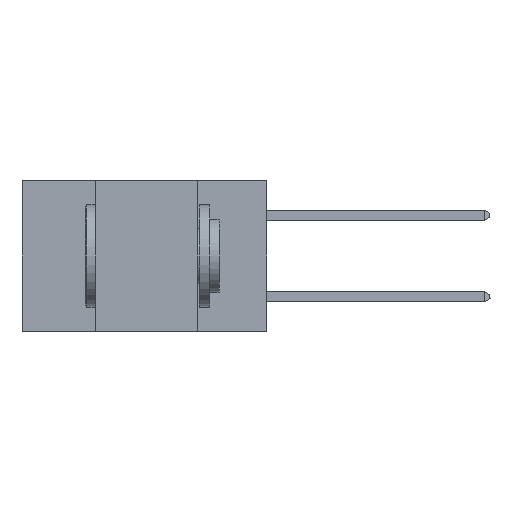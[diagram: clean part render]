
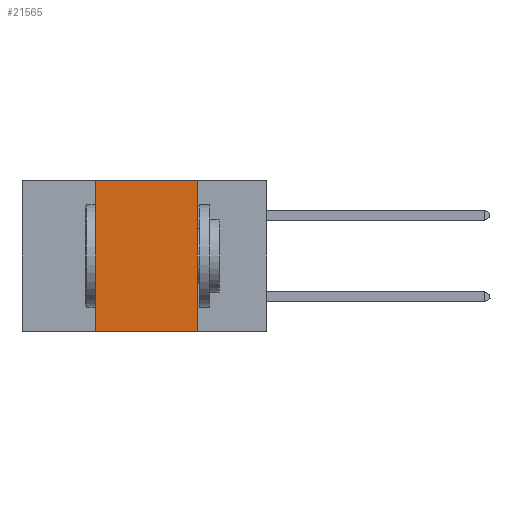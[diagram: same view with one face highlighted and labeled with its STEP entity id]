
A CAD part, left-side view. The second image highlights one B-rep face of the part: STEP entity #21565.
In plain terms, the highlighted planar face has unit normal (-1, 0, 0).
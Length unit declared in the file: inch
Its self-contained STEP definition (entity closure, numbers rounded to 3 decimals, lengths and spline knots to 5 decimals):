
#768 = DIRECTION ( 'NONE',  ( 0., -1., 0. ) ) ;
#1853 = VECTOR ( 'NONE', #768, 39.37008 ) ;
#1929 = ORIENTED_EDGE ( 'NONE', *, *, #16639, .F. ) ;
#1976 = LINE ( 'NONE', #21147, #2717 ) ;
#2556 = VERTEX_POINT ( 'NONE', #9746 ) ;
#2717 = VECTOR ( 'NONE', #15711, 39.37008 ) ;
#3177 = EDGE_CURVE ( 'NONE', #22099, #7793, #5542, .T. ) ;
#3540 = CARTESIAN_POINT ( 'NONE',  ( 0., 0.17, -0.37 ) ) ;
#3684 = LINE ( 'NONE', #7576, #5959 ) ;
#4507 = FACE_OUTER_BOUND ( 'NONE', #18668, .T. ) ;
#5542 = LINE ( 'NONE', #13347, #1853 ) ;
#5700 = CARTESIAN_POINT ( 'NONE',  ( 0., 0.6, 0. ) ) ;
#5959 = VECTOR ( 'NONE', #20226, 39.37008 ) ;
#6013 = DIRECTION ( 'NONE',  ( 0., 0., -1. ) ) ;
#7150 = VECTOR ( 'NONE', #7552, 39.37008 ) ;
#7552 = DIRECTION ( 'NONE',  ( 0., 0., 1. ) ) ;
#7576 = CARTESIAN_POINT ( 'NONE',  ( 0., 0.17, 0. ) ) ;
#7793 = VERTEX_POINT ( 'NONE', #3540 ) ;
#8451 = EDGE_CURVE ( 'NONE', #2556, #7793, #3684, .T. ) ;
#9746 = CARTESIAN_POINT ( 'NONE',  ( 0., 0.17, 0. ) ) ;
#10593 = ORIENTED_EDGE ( 'NONE', *, *, #3177, .T. ) ;
#10603 = CARTESIAN_POINT ( 'NONE',  ( 0., 0.42, -0.37 ) ) ;
#10782 = ORIENTED_EDGE ( 'NONE', *, *, #8451, .F. ) ;
#12579 = PLANE ( 'NONE',  #18594 ) ;
#13347 = CARTESIAN_POINT ( 'NONE',  ( 0., 0.6, -0.37 ) ) ;
#13419 = EDGE_CURVE ( 'NONE', #20018, #2556, #1976, .T. ) ;
#14226 = LINE ( 'NONE', #20042, #7150 ) ;
#14494 = ORIENTED_EDGE ( 'NONE', *, *, #13419, .F. ) ;
#15711 = DIRECTION ( 'NONE',  ( 0., -1., 0. ) ) ;
#16639 = EDGE_CURVE ( 'NONE', #22099, #20018, #14226, .T. ) ;
#16761 = DIRECTION ( 'NONE',  ( 1., 0., 0. ) ) ;
#18594 = AXIS2_PLACEMENT_3D ( 'NONE', #5700, #16761, #6013 ) ;
#18668 = EDGE_LOOP ( 'NONE', ( #10782, #14494, #1929, #10593 ) ) ;
#19514 = CARTESIAN_POINT ( 'NONE',  ( 0., 0.42, 0. ) ) ;
#20018 = VERTEX_POINT ( 'NONE', #19514 ) ;
#20042 = CARTESIAN_POINT ( 'NONE',  ( 0., 0.42, 0. ) ) ;
#20226 = DIRECTION ( 'NONE',  ( 0., 0., -1. ) ) ;
#21147 = CARTESIAN_POINT ( 'NONE',  ( 0., 0.6, 0. ) ) ;
#21565 = ADVANCED_FACE ( 'NONE', ( #4507 ), #12579, .F. ) ;
#22099 = VERTEX_POINT ( 'NONE', #10603 ) ;
